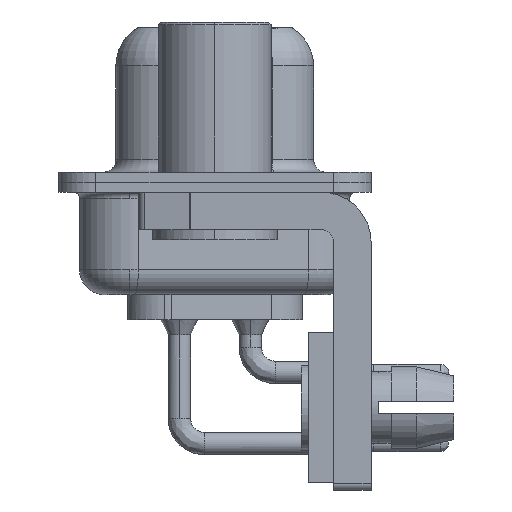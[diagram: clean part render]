
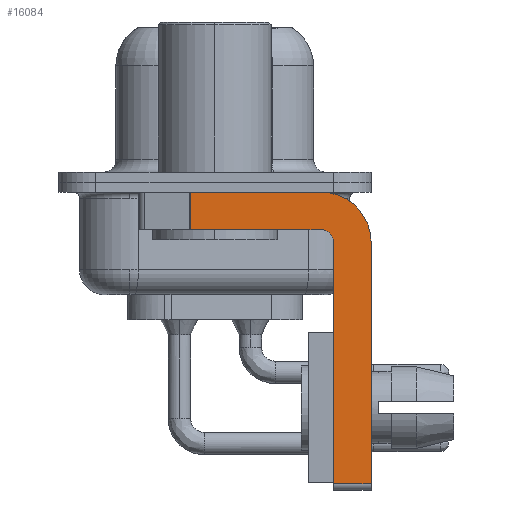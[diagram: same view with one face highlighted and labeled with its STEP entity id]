
A CAD part, left-side view. The second image highlights one B-rep face of the part: STEP entity #16084.
In plain terms, the highlighted planar face has unit normal (-1, 0, 0).
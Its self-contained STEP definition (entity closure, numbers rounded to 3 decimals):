
#786 = VERTEX_POINT ( 'NONE', #19783 ) ;
#1119 = CARTESIAN_POINT ( 'NONE',  ( -2.9, -4.25, -2.4 ) ) ;
#1254 = VERTEX_POINT ( 'NONE', #2885 ) ;
#1990 = DIRECTION ( 'NONE',  ( 0., 0., 1. ) ) ;
#2047 = ORIENTED_EDGE ( 'NONE', *, *, #5221, .T. ) ;
#2206 = EDGE_CURVE ( 'NONE', #23092, #27804, #17533, .T. ) ;
#2491 = VECTOR ( 'NONE', #10797, 1000. ) ;
#2885 = CARTESIAN_POINT ( 'NONE',  ( -2.9, -4.25, -1.9 ) ) ;
#2934 = DIRECTION ( 'NONE',  ( 0., 1., 0. ) ) ;
#3191 = ORIENTED_EDGE ( 'NONE', *, *, #18339, .F. ) ;
#3209 = CARTESIAN_POINT ( 'NONE',  ( -2.9, 0.978, -1.9 ) ) ;
#3832 = DIRECTION ( 'NONE',  ( 0., 0., -1. ) ) ;
#4388 = ORIENTED_EDGE ( 'NONE', *, *, #27485, .F. ) ;
#4541 = LINE ( 'NONE', #30145, #30945 ) ;
#5221 = EDGE_CURVE ( 'NONE', #786, #22739, #18426, .T. ) ;
#5427 = DIRECTION ( 'NONE',  ( 1., 0., 0. ) ) ;
#6398 = EDGE_LOOP ( 'NONE', ( #8947, #2047, #21280, #8761, #4388, #9556, #14611, #3191 ) ) ;
#7357 = AXIS2_PLACEMENT_3D ( 'NONE', #1119, #19270, #3832 ) ;
#8191 = CARTESIAN_POINT ( 'NONE',  ( -2.9, -4.25, -1.9 ) ) ;
#8761 = ORIENTED_EDGE ( 'NONE', *, *, #23578, .F. ) ;
#8947 = ORIENTED_EDGE ( 'NONE', *, *, #18516, .F. ) ;
#8995 = CARTESIAN_POINT ( 'NONE',  ( -2.9, -6.25, -12.05 ) ) ;
#9457 = CIRCLE ( 'NONE', #7357, 2. ) ;
#9556 = ORIENTED_EDGE ( 'NONE', *, *, #11795, .T. ) ;
#10797 = DIRECTION ( 'NONE',  ( 0., -1., 0. ) ) ;
#11705 = VECTOR ( 'NONE', #29993, 1000. ) ;
#11795 = EDGE_CURVE ( 'NONE', #29865, #27804, #23860, .T. ) ;
#12218 = LINE ( 'NONE', #8191, #31697 ) ;
#12748 = DIRECTION ( 'NONE',  ( 0., 0., 1. ) ) ;
#13355 = AXIS2_PLACEMENT_3D ( 'NONE', #20759, #5427, #23323 ) ;
#13648 = VERTEX_POINT ( 'NONE', #29218 ) ;
#14611 = ORIENTED_EDGE ( 'NONE', *, *, #2206, .F. ) ;
#15540 = VERTEX_POINT ( 'NONE', #28430 ) ;
#16084 = ADVANCED_FACE ( 'NONE', ( #16096 ), #25699, .F. ) ;
#16096 = FACE_OUTER_BOUND ( 'NONE', #6398, .T. ) ;
#17533 = LINE ( 'NONE', #22533, #29437 ) ;
#17559 = DIRECTION ( 'NONE',  ( -1., 0., 0. ) ) ;
#18339 = EDGE_CURVE ( 'NONE', #15540, #23092, #9457, .T. ) ;
#18426 = LINE ( 'NONE', #30029, #11705 ) ;
#18516 = EDGE_CURVE ( 'NONE', #786, #15540, #4541, .T. ) ;
#19154 = DIRECTION ( 'NONE',  ( 0., 0., -1. ) ) ;
#19270 = DIRECTION ( 'NONE',  ( 1., 0., 0. ) ) ;
#19783 = CARTESIAN_POINT ( 'NONE',  ( -2.9, 0.978, -0.4 ) ) ;
#20050 = DIRECTION ( 'NONE',  ( 0., -1., 0. ) ) ;
#20759 = CARTESIAN_POINT ( 'NONE',  ( -2.9, -4.25, -2.4 ) ) ;
#21280 = ORIENTED_EDGE ( 'NONE', *, *, #26909, .F. ) ;
#22533 = CARTESIAN_POINT ( 'NONE',  ( -2.9, -6.25, -2.4 ) ) ;
#22739 = VERTEX_POINT ( 'NONE', #3209 ) ;
#23092 = VERTEX_POINT ( 'NONE', #30224 ) ;
#23323 = DIRECTION ( 'NONE',  ( 0., 0., -1. ) ) ;
#23578 = EDGE_CURVE ( 'NONE', #13648, #1254, #26192, .T. ) ;
#23860 = LINE ( 'NONE', #25945, #2491 ) ;
#24815 = LINE ( 'NONE', #25294, #31660 ) ;
#25294 = CARTESIAN_POINT ( 'NONE',  ( -2.9, -4.75, -12.3 ) ) ;
#25699 = PLANE ( 'NONE',  #13355 ) ;
#25945 = CARTESIAN_POINT ( 'NONE',  ( -2.9, -4.25, -12.05 ) ) ;
#26192 = CIRCLE ( 'NONE', #28148, 0.5 ) ;
#26909 = EDGE_CURVE ( 'NONE', #1254, #22739, #12218, .T. ) ;
#27485 = EDGE_CURVE ( 'NONE', #29865, #13648, #24815, .T. ) ;
#27804 = VERTEX_POINT ( 'NONE', #8995 ) ;
#28148 = AXIS2_PLACEMENT_3D ( 'NONE', #32822, #17559, #1990 ) ;
#28430 = CARTESIAN_POINT ( 'NONE',  ( -2.9, -4.25, -0.4 ) ) ;
#29218 = CARTESIAN_POINT ( 'NONE',  ( -2.9, -4.75, -2.4 ) ) ;
#29437 = VECTOR ( 'NONE', #19154, 1000. ) ;
#29865 = VERTEX_POINT ( 'NONE', #31227 ) ;
#29993 = DIRECTION ( 'NONE',  ( 0., 0., -1. ) ) ;
#30029 = CARTESIAN_POINT ( 'NONE',  ( -2.9, 0.978, -1.9 ) ) ;
#30145 = CARTESIAN_POINT ( 'NONE',  ( -2.9, 3., -0.4 ) ) ;
#30224 = CARTESIAN_POINT ( 'NONE',  ( -2.9, -6.25, -2.4 ) ) ;
#30945 = VECTOR ( 'NONE', #20050, 1000. ) ;
#31227 = CARTESIAN_POINT ( 'NONE',  ( -2.9, -4.75, -12.05 ) ) ;
#31660 = VECTOR ( 'NONE', #12748, 1000. ) ;
#31697 = VECTOR ( 'NONE', #2934, 1000. ) ;
#32822 = CARTESIAN_POINT ( 'NONE',  ( -2.9, -4.25, -2.4 ) ) ;
